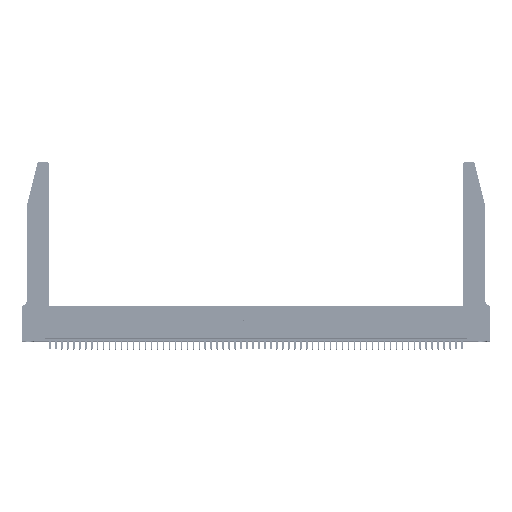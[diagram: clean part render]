
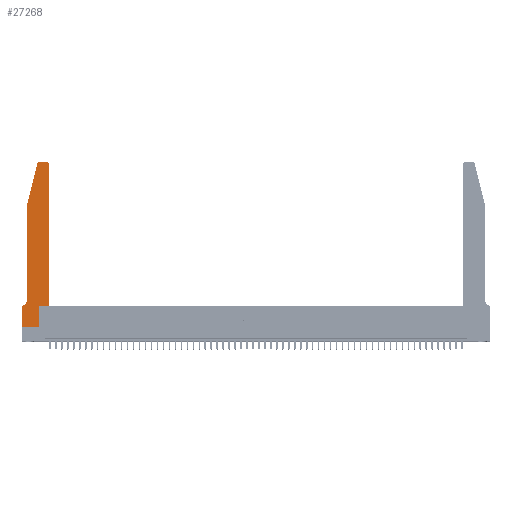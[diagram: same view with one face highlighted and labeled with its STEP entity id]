
A CAD part, top view. The second image highlights one B-rep face of the part: STEP entity #27268.
In plain terms, the highlighted planar face has unit normal (0, 0, 1).
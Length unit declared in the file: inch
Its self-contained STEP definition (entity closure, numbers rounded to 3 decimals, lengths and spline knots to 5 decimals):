
#404 = DIRECTION ( 'NONE',  ( 0., 1., 0. ) ) ;
#414 = CARTESIAN_POINT ( 'NONE',  ( 0.2865, 0., 0.37 ) ) ;
#2083 = EDGE_CURVE ( 'NONE', #53368, #7168, #23115, .T. ) ;
#2237 = CARTESIAN_POINT ( 'NONE',  ( 0., 0.35, 0.37 ) ) ;
#3168 = CARTESIAN_POINT ( 'NONE',  ( 0., 0., 0.37 ) ) ;
#3599 = EDGE_CURVE ( 'NONE', #10484, #52763, #30308, .T. ) ;
#3739 = CARTESIAN_POINT ( 'NONE',  ( 0.2605, 2.75, 0.37 ) ) ;
#4496 = EDGE_CURVE ( 'NONE', #44275, #38860, #41724, .T. ) ;
#5669 = CARTESIAN_POINT ( 'NONE',  ( 0.0055, 0.42, 0.37 ) ) ;
#5681 = ORIENTED_EDGE ( 'NONE', *, *, #24461, .T. ) ;
#6924 = VERTEX_POINT ( 'NONE', #33931 ) ;
#7168 = VERTEX_POINT ( 'NONE', #47632 ) ;
#7812 = CARTESIAN_POINT ( 'NONE',  ( 0.4505, 0.35, 0.37 ) ) ;
#7927 = CARTESIAN_POINT ( 'NONE',  ( 0., 0., 0.37 ) ) ;
#7989 = VERTEX_POINT ( 'NONE', #52959 ) ;
#10013 = CARTESIAN_POINT ( 'NONE',  ( 0.4205, 2.75, 0.37 ) ) ;
#10069 = DIRECTION ( 'NONE',  ( -1., 0., 0. ) ) ;
#10181 = EDGE_LOOP ( 'NONE', ( #37863, #20133, #24583, #30187, #15536, #47349, #12393, #49896, #48441, #44090, #5681, #22762 ) ) ;
#10484 = VERTEX_POINT ( 'NONE', #414 ) ;
#10621 = CARTESIAN_POINT ( 'NONE',  ( 0.0055, 0.35, 0.37 ) ) ;
#11635 = VECTOR ( 'NONE', #42659, 39.37008 ) ;
#11800 = CARTESIAN_POINT ( 'NONE',  ( 0.2865, 0.35, 0.37 ) ) ;
#12296 = DIRECTION ( 'NONE',  ( 0., -1., 0. ) ) ;
#12393 = ORIENTED_EDGE ( 'NONE', *, *, #23618, .T. ) ;
#13094 = LINE ( 'NONE', #55633, #23190 ) ;
#13640 = CARTESIAN_POINT ( 'NONE',  ( 0.4205, 2.72, 0.37 ) ) ;
#15380 = DIRECTION ( 'NONE',  ( 0., 0., 1. ) ) ;
#15536 = ORIENTED_EDGE ( 'NONE', *, *, #54992, .T. ) ;
#15976 = CARTESIAN_POINT ( 'NONE',  ( 0.0755, 0.35, 0.37 ) ) ;
#17574 = VECTOR ( 'NONE', #404, 39.37008 ) ;
#17992 = DIRECTION ( 'NONE',  ( 1., 0., 0. ) ) ;
#18245 = EDGE_CURVE ( 'NONE', #48318, #10484, #13094, .T. ) ;
#18982 = LINE ( 'NONE', #52052, #40556 ) ;
#19530 = EDGE_CURVE ( 'NONE', #52763, #36617, #18982, .T. ) ;
#20133 = ORIENTED_EDGE ( 'NONE', *, *, #2083, .T. ) ;
#20514 = VECTOR ( 'NONE', #46110, 39.37008 ) ;
#20602 = VECTOR ( 'NONE', #12296, 39.37008 ) ;
#21197 = DIRECTION ( 'NONE',  ( 1., 0., 0. ) ) ;
#21257 = LINE ( 'NONE', #28725, #31329 ) ;
#21641 = CARTESIAN_POINT ( 'NONE',  ( 0.284, 2.72, 0.37 ) ) ;
#22344 = CARTESIAN_POINT ( 'NONE',  ( 0.0755, 0.42, 0.37 ) ) ;
#22762 = ORIENTED_EDGE ( 'NONE', *, *, #4496, .T. ) ;
#23094 = AXIS2_PLACEMENT_3D ( 'NONE', #2237, #15380, #45535 ) ;
#23115 = CIRCLE ( 'NONE', #51373, 0.03 ) ;
#23190 = VECTOR ( 'NONE', #21197, 39.37008 ) ;
#23618 = EDGE_CURVE ( 'NONE', #7989, #48318, #43533, .T. ) ;
#24404 = DIRECTION ( 'NONE',  ( 0., -1., 0. ) ) ;
#24423 = LINE ( 'NONE', #3739, #11635 ) ;
#24461 = EDGE_CURVE ( 'NONE', #36617, #44275, #28570, .T. ) ;
#24583 = ORIENTED_EDGE ( 'NONE', *, *, #52415, .T. ) ;
#24797 = EDGE_CURVE ( 'NONE', #6924, #40061, #21257, .T. ) ;
#25089 = FACE_OUTER_BOUND ( 'NONE', #10181, .T. ) ;
#25280 = AXIS2_PLACEMENT_3D ( 'NONE', #5669, #35874, #10069 ) ;
#25963 = DIRECTION ( 'NONE',  ( 1., 0., 0. ) ) ;
#25986 = CIRCLE ( 'NONE', #25280, 0.07 ) ;
#26121 = CARTESIAN_POINT ( 'NONE',  ( 0.0755, 2., 0.37 ) ) ;
#26297 = DIRECTION ( 'NONE',  ( -0.239, -0.971, 0. ) ) ;
#27268 = ADVANCED_FACE ( 'NONE', ( #25089 ), #41190, .T. ) ;
#27537 = VECTOR ( 'NONE', #26297, 39.37008 ) ;
#28570 = LINE ( 'NONE', #48203, #46143 ) ;
#28725 = CARTESIAN_POINT ( 'NONE',  ( 0.0755, 2., 0.37 ) ) ;
#30187 = ORIENTED_EDGE ( 'NONE', *, *, #24797, .T. ) ;
#30308 = LINE ( 'NONE', #52157, #17574 ) ;
#31329 = VECTOR ( 'NONE', #24404, 39.37008 ) ;
#32740 = VERTEX_POINT ( 'NONE', #10621 ) ;
#33931 = CARTESIAN_POINT ( 'NONE',  ( 0.0755, 2., 0.37 ) ) ;
#35874 = DIRECTION ( 'NONE',  ( 0., 0., -1. ) ) ;
#36617 = VERTEX_POINT ( 'NONE', #7812 ) ;
#37863 = ORIENTED_EDGE ( 'NONE', *, *, #48410, .T. ) ;
#38100 = AXIS2_PLACEMENT_3D ( 'NONE', #13640, #43799, #17992 ) ;
#38860 = VERTEX_POINT ( 'NONE', #10013 ) ;
#39542 = DIRECTION ( 'NONE',  ( 0., 1., 0. ) ) ;
#40061 = VERTEX_POINT ( 'NONE', #22344 ) ;
#40412 = LINE ( 'NONE', #26121, #27537 ) ;
#40556 = VECTOR ( 'NONE', #47781, 39.37008 ) ;
#41190 = PLANE ( 'NONE',  #23094 ) ;
#41724 = CIRCLE ( 'NONE', #38100, 0.03 ) ;
#42659 = DIRECTION ( 'NONE',  ( -1., 0., 0. ) ) ;
#43140 = EDGE_CURVE ( 'NONE', #32740, #7989, #50809, .T. ) ;
#43533 = LINE ( 'NONE', #7927, #20602 ) ;
#43799 = DIRECTION ( 'NONE',  ( 0., 0., 1. ) ) ;
#44090 = ORIENTED_EDGE ( 'NONE', *, *, #19530, .T. ) ;
#44275 = VERTEX_POINT ( 'NONE', #53845 ) ;
#45535 = DIRECTION ( 'NONE',  ( 1., 0., 0. ) ) ;
#46110 = DIRECTION ( 'NONE',  ( -1., 0., 0. ) ) ;
#46143 = VECTOR ( 'NONE', #39542, 39.37008 ) ;
#46429 = CARTESIAN_POINT ( 'NONE',  ( 0.284, 2.75, 0.37 ) ) ;
#47349 = ORIENTED_EDGE ( 'NONE', *, *, #43140, .T. ) ;
#47632 = CARTESIAN_POINT ( 'NONE',  ( 0.25487, 2.72718, 0.37 ) ) ;
#47781 = DIRECTION ( 'NONE',  ( 1., 0., 0. ) ) ;
#48203 = CARTESIAN_POINT ( 'NONE',  ( 0.4505, 0.35, 0.37 ) ) ;
#48318 = VERTEX_POINT ( 'NONE', #3168 ) ;
#48410 = EDGE_CURVE ( 'NONE', #38860, #53368, #24423, .T. ) ;
#48441 = ORIENTED_EDGE ( 'NONE', *, *, #3599, .T. ) ;
#49896 = ORIENTED_EDGE ( 'NONE', *, *, #18245, .T. ) ;
#50809 = LINE ( 'NONE', #15976, #20514 ) ;
#51373 = AXIS2_PLACEMENT_3D ( 'NONE', #21641, #51752, #25963 ) ;
#51752 = DIRECTION ( 'NONE',  ( 0., 0., 1. ) ) ;
#52052 = CARTESIAN_POINT ( 'NONE',  ( 0.4505, 0.35, 0.37 ) ) ;
#52157 = CARTESIAN_POINT ( 'NONE',  ( 0.2865, 0.35, 0.37 ) ) ;
#52415 = EDGE_CURVE ( 'NONE', #7168, #6924, #40412, .T. ) ;
#52763 = VERTEX_POINT ( 'NONE', #11800 ) ;
#52959 = CARTESIAN_POINT ( 'NONE',  ( 0., 0.35, 0.37 ) ) ;
#53368 = VERTEX_POINT ( 'NONE', #46429 ) ;
#53845 = CARTESIAN_POINT ( 'NONE',  ( 0.4505, 2.72, 0.37 ) ) ;
#54992 = EDGE_CURVE ( 'NONE', #40061, #32740, #25986, .T. ) ;
#55633 = CARTESIAN_POINT ( 'NONE',  ( 0., 0., 0.37 ) ) ;
